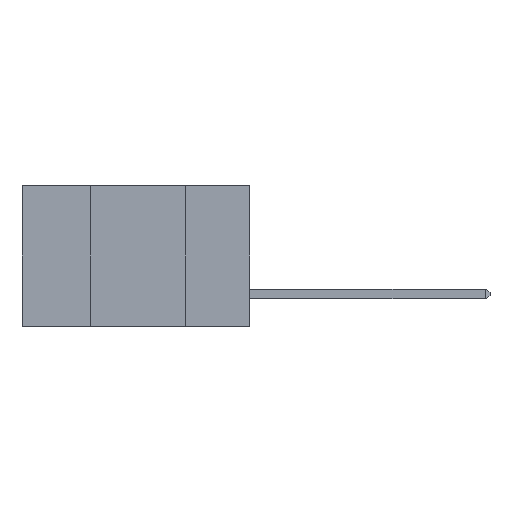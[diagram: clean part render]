
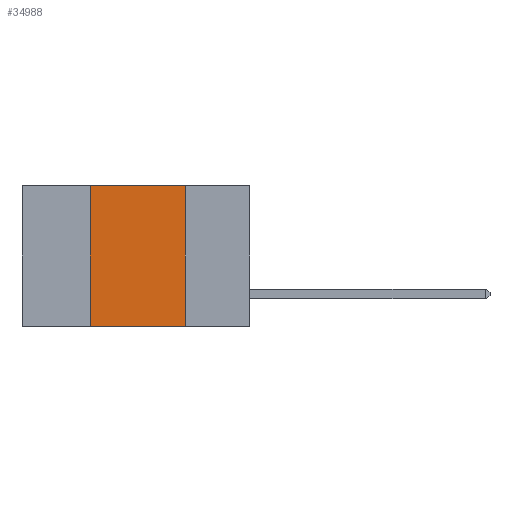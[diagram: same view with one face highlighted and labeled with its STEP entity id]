
A CAD part, left-side view. The second image highlights one B-rep face of the part: STEP entity #34988.
In plain terms, the highlighted planar face has unit normal (-1, 0, 0).
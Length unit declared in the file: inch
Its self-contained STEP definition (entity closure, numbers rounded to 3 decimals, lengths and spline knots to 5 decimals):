
#588 = VERTEX_POINT ( 'NONE', #6594 ) ;
#1236 = FACE_OUTER_BOUND ( 'NONE', #4662, .T. ) ;
#1277 = CARTESIAN_POINT ( 'NONE',  ( 0., 0.42, -0.37 ) ) ;
#1417 = DIRECTION ( 'NONE',  ( 0., -1., 0. ) ) ;
#4055 = DIRECTION ( 'NONE',  ( 0., -1., 0. ) ) ;
#4113 = VERTEX_POINT ( 'NONE', #37152 ) ;
#4662 = EDGE_LOOP ( 'NONE', ( #32883, #23482, #36000, #5435 ) ) ;
#5146 = VECTOR ( 'NONE', #24868, 39.37008 ) ;
#5433 = CARTESIAN_POINT ( 'NONE',  ( 0., 0.6, 0. ) ) ;
#5435 = ORIENTED_EDGE ( 'NONE', *, *, #21981, .T. ) ;
#6594 = CARTESIAN_POINT ( 'NONE',  ( 0., 0.17, -0.37 ) ) ;
#9835 = EDGE_CURVE ( 'NONE', #27189, #588, #24546, .T. ) ;
#11004 = LINE ( 'NONE', #24508, #32895 ) ;
#14252 = PLANE ( 'NONE',  #28596 ) ;
#14783 = CARTESIAN_POINT ( 'NONE',  ( 0., 0.17, 0. ) ) ;
#17142 = DIRECTION ( 'NONE',  ( 1., 0., 0. ) ) ;
#19027 = VECTOR ( 'NONE', #4055, 39.37008 ) ;
#19044 = EDGE_CURVE ( 'NONE', #26786, #4113, #20552, .T. ) ;
#20143 = CARTESIAN_POINT ( 'NONE',  ( 0., 0.17, 0. ) ) ;
#20552 = LINE ( 'NONE', #22032, #5146 ) ;
#21981 = EDGE_CURVE ( 'NONE', #26786, #588, #26555, .T. ) ;
#22032 = CARTESIAN_POINT ( 'NONE',  ( 0., 0.42, 0. ) ) ;
#23482 = ORIENTED_EDGE ( 'NONE', *, *, #29954, .F. ) ;
#24508 = CARTESIAN_POINT ( 'NONE',  ( 0., 0.6, 0. ) ) ;
#24546 = LINE ( 'NONE', #20143, #32185 ) ;
#24868 = DIRECTION ( 'NONE',  ( 0., 0., 1. ) ) ;
#26555 = LINE ( 'NONE', #35607, #19027 ) ;
#26786 = VERTEX_POINT ( 'NONE', #1277 ) ;
#27189 = VERTEX_POINT ( 'NONE', #14783 ) ;
#28596 = AXIS2_PLACEMENT_3D ( 'NONE', #5433, #17142, #37105 ) ;
#29954 = EDGE_CURVE ( 'NONE', #4113, #27189, #11004, .T. ) ;
#32185 = VECTOR ( 'NONE', #37225, 39.37008 ) ;
#32883 = ORIENTED_EDGE ( 'NONE', *, *, #9835, .F. ) ;
#32895 = VECTOR ( 'NONE', #1417, 39.37008 ) ;
#34988 = ADVANCED_FACE ( 'NONE', ( #1236 ), #14252, .F. ) ;
#35607 = CARTESIAN_POINT ( 'NONE',  ( 0., 0.6, -0.37 ) ) ;
#36000 = ORIENTED_EDGE ( 'NONE', *, *, #19044, .F. ) ;
#37105 = DIRECTION ( 'NONE',  ( 0., 0., -1. ) ) ;
#37152 = CARTESIAN_POINT ( 'NONE',  ( 0., 0.42, 0. ) ) ;
#37225 = DIRECTION ( 'NONE',  ( 0., 0., -1. ) ) ;
